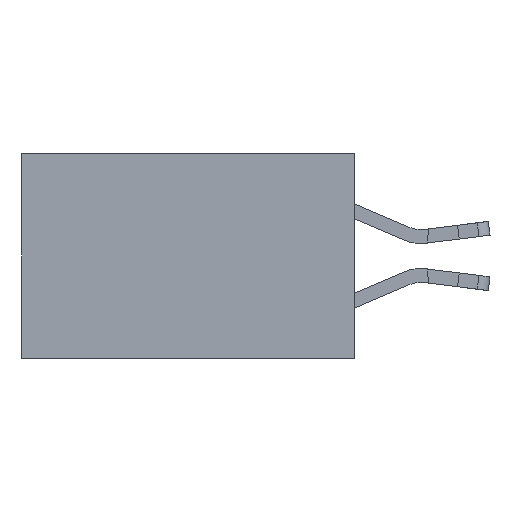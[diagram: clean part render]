
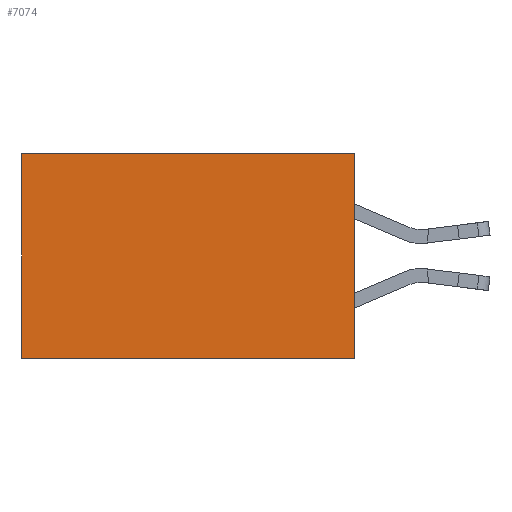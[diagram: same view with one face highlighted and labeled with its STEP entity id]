
A CAD part, left-side view. The second image highlights one B-rep face of the part: STEP entity #7074.
In plain terms, the highlighted planar face has unit normal (-1, 0, 0).
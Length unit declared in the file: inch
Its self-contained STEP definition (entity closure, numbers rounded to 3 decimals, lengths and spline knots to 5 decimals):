
#702 = PLANE ( 'NONE',  #13109 ) ;
#1040 = DIRECTION ( 'NONE',  ( 0., 0., -1. ) ) ;
#1210 = DIRECTION ( 'NONE',  ( 0., 0., -1. ) ) ;
#1306 = ORIENTED_EDGE ( 'NONE', *, *, #4544, .T. ) ;
#1427 = LINE ( 'NONE', #8772, #10089 ) ;
#2437 = DIRECTION ( 'NONE',  ( 1., 0., 0. ) ) ;
#2620 = CARTESIAN_POINT ( 'NONE',  ( 0.298, 0., 0. ) ) ;
#2761 = CARTESIAN_POINT ( 'NONE',  ( 0.298, 0., 0. ) ) ;
#2814 = DIRECTION ( 'NONE',  ( 0., 0., -1. ) ) ;
#2834 = CARTESIAN_POINT ( 'NONE',  ( 0.298, 0.6, 0. ) ) ;
#3528 = ORIENTED_EDGE ( 'NONE', *, *, #5561, .F. ) ;
#3716 = VERTEX_POINT ( 'NONE', #2620 ) ;
#4023 = LINE ( 'NONE', #7589, #13174 ) ;
#4544 = EDGE_CURVE ( 'NONE', #3716, #9902, #13426, .T. ) ;
#4640 = CARTESIAN_POINT ( 'NONE',  ( 0.298, 0., -0.37 ) ) ;
#4729 = EDGE_CURVE ( 'NONE', #13388, #6992, #4023, .T. ) ;
#5456 = VECTOR ( 'NONE', #1040, 39.37008 ) ;
#5561 = EDGE_CURVE ( 'NONE', #3716, #13388, #1427, .T. ) ;
#6992 = VERTEX_POINT ( 'NONE', #11794 ) ;
#7074 = ADVANCED_FACE ( 'NONE', ( #13814 ), #702, .F. ) ;
#7241 = EDGE_CURVE ( 'NONE', #9902, #6992, #11319, .T. ) ;
#7538 = EDGE_LOOP ( 'NONE', ( #12084, #9723, #3528, #1306 ) ) ;
#7589 = CARTESIAN_POINT ( 'NONE',  ( 0.298, 0., -0.37 ) ) ;
#7629 = DIRECTION ( 'NONE',  ( 0., 1., 0. ) ) ;
#8772 = CARTESIAN_POINT ( 'NONE',  ( 0.298, 0., 0. ) ) ;
#9482 = CARTESIAN_POINT ( 'NONE',  ( 0.298, 0., 0. ) ) ;
#9548 = CARTESIAN_POINT ( 'NONE',  ( 0.298, 0.6, 0. ) ) ;
#9585 = DIRECTION ( 'NONE',  ( 0., 1., 0. ) ) ;
#9723 = ORIENTED_EDGE ( 'NONE', *, *, #4729, .F. ) ;
#9902 = VERTEX_POINT ( 'NONE', #2834 ) ;
#10089 = VECTOR ( 'NONE', #1210, 39.37008 ) ;
#11319 = LINE ( 'NONE', #9548, #5456 ) ;
#11794 = CARTESIAN_POINT ( 'NONE',  ( 0.298, 0.6, -0.37 ) ) ;
#12084 = ORIENTED_EDGE ( 'NONE', *, *, #7241, .T. ) ;
#13070 = VECTOR ( 'NONE', #9585, 39.37008 ) ;
#13109 = AXIS2_PLACEMENT_3D ( 'NONE', #2761, #2437, #2814 ) ;
#13174 = VECTOR ( 'NONE', #7629, 39.37008 ) ;
#13388 = VERTEX_POINT ( 'NONE', #4640 ) ;
#13426 = LINE ( 'NONE', #9482, #13070 ) ;
#13814 = FACE_OUTER_BOUND ( 'NONE', #7538, .T. ) ;
